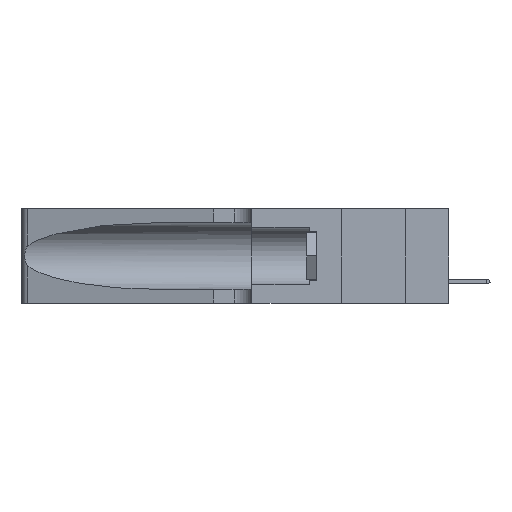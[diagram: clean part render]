
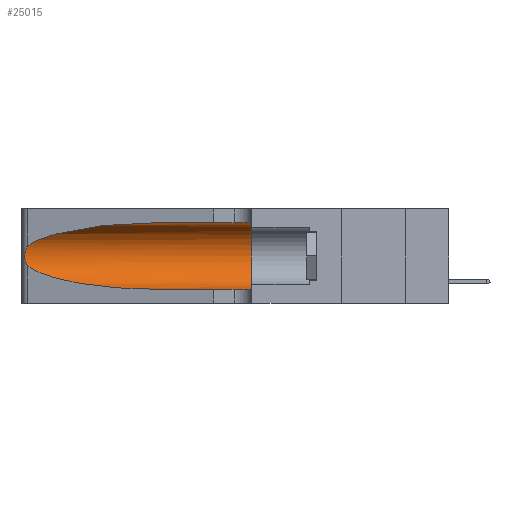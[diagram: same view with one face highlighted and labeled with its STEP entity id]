
A CAD part, left-side view. The second image highlights one B-rep face of the part: STEP entity #25015.
In plain terms, the highlighted cylindrical face has radius 3.308 mm (diameter 6.617 mm), a partial arc.
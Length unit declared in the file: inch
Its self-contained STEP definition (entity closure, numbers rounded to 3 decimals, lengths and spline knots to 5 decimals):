
#1150 = CARTESIAN_POINT ( 'NONE',  ( 0.25639, 1.23186, 0.15144 ) ) ;
#1614 = CARTESIAN_POINT ( 'NONE',  ( 0.25789, 1.23486, 0.15765 ) ) ;
#3197 = VERTEX_POINT ( 'NONE', #30987 ) ;
#4556 = CARTESIAN_POINT ( 'NONE',  ( 0.25639, 1.23184, 0.21858 ) ) ;
#4716 = CARTESIAN_POINT ( 'NONE',  ( 0.25487, 1.22718, 0.22369 ) ) ;
#4862 = CARTESIAN_POINT ( 'NONE',  ( 0.25854, 1.2359, 0.20912 ) ) ;
#5605 = ORIENTED_EDGE ( 'NONE', *, *, #19120, .T. ) ;
#5945 = ORIENTED_EDGE ( 'NONE', *, *, #38050, .T. ) ;
#5971 = EDGE_CURVE ( 'NONE', #21398, #3197, #44074, .T. ) ;
#7481 = EDGE_CURVE ( 'NONE', #19406, #3197, #38464, .T. ) ;
#7937 = CARTESIAN_POINT ( 'NONE',  ( 0.1305, 0.35, 0.31525 ) ) ;
#8434 = CARTESIAN_POINT ( 'NONE',  ( 0.26075, 1.23896, 0.19203 ) ) ;
#8736 = CARTESIAN_POINT ( 'NONE',  ( 0.25487, 1.22718, 0.14631 ) ) ;
#9208 = CARTESIAN_POINT ( 'NONE',  ( 0.25487, 1.22718, 0.22369 ) ) ;
#9624 = DIRECTION ( 'NONE',  ( 0., 0., 1. ) ) ;
#11632 = CARTESIAN_POINT ( 'NONE',  ( 0.1305, 0.72297, 0.31525 ) ) ;
#12654 = DIRECTION ( 'NONE',  ( 0., 0., -1. ) ) ;
#13403 = AXIS2_PLACEMENT_3D ( 'NONE', #30616, #40782, #9624 ) ;
#16372 = CARTESIAN_POINT ( 'NONE',  ( 0.1305, 1.61858, 0.05475 ) ) ;
#17282 = CARTESIAN_POINT ( 'NONE',  ( 0.2373, 1.15595, 0.28018 ) ) ;
#17976 = CARTESIAN_POINT ( 'NONE',  ( 0.1305, 1.61858, 0.31525 ) ) ;
#18551 = VECTOR ( 'NONE', #30289, 39.37008 ) ;
#19120 = EDGE_CURVE ( 'NONE', #34291, #19406, #44472, .T. ) ;
#19217 = CARTESIAN_POINT ( 'NONE',  ( 0.26017, 1.23833, 0.17102 ) ) ;
#19406 = VERTEX_POINT ( 'NONE', #29767 ) ;
#19437 = CARTESIAN_POINT ( 'NONE',  ( 0.18966, 0.96281, 0.05475 ) ) ;
#20327 = DIRECTION ( 'NONE',  ( 0., -1., 0. ) ) ;
#21398 = VERTEX_POINT ( 'NONE', #7937 ) ;
#21823 = EDGE_CURVE ( 'NONE', #23246, #34291, #42988, .T. ) ;
#22641 = CARTESIAN_POINT ( 'NONE',  ( 0.25555, 1.22994, 0.2215 ) ) ;
#22698 = CARTESIAN_POINT ( 'NONE',  ( 0.1305, 0.72297, 0.05475 ) ) ;
#22807 = CARTESIAN_POINT ( 'NONE',  ( 0.25856, 1.23593, 0.16098 ) ) ;
#23246 = VERTEX_POINT ( 'NONE', #9208 ) ;
#25015 = ADVANCED_FACE ( 'NONE', ( #35313 ), #33100, .F. ) ;
#26240 = CARTESIAN_POINT ( 'NONE',  ( 0.25487, 1.22718, 0.14631 ) ) ;
#26338 = CARTESIAN_POINT ( 'NONE',  ( 0.25555, 1.22993, 0.14849 ) ) ;
#26874 = CARTESIAN_POINT ( 'NONE',  ( 0.2373, 1.15595, 0.08982 ) ) ;
#27205 = CARTESIAN_POINT ( 'NONE',  ( 0.1305, 1.61858, 0.185 ) ) ;
#27216 = VERTEX_POINT ( 'NONE', #11632 ) ;
#28097 = CARTESIAN_POINT ( 'NONE',  ( 0.25487, 1.22718, 0.22369 ) ) ;
#29767 = CARTESIAN_POINT ( 'NONE',  ( 0.1305, 0.72297, 0.05475 ) ) ;
#30289 = DIRECTION ( 'NONE',  ( 0., -1., 0. ) ) ;
#30616 = CARTESIAN_POINT ( 'NONE',  ( 0.1305, 0.35, 0.185 ) ) ;
#30975 = ORIENTED_EDGE ( 'NONE', *, *, #7481, .T. ) ;
#30987 = CARTESIAN_POINT ( 'NONE',  ( 0.1305, 0.35, 0.05475 ) ) ;
#31242 = EDGE_CURVE ( 'NONE', #27216, #21398, #35997, .T. ) ;
#31627 = VECTOR ( 'NONE', #20327, 39.37008 ) ;
#32450 = ORIENTED_EDGE ( 'NONE', *, *, #5971, .F. ) ;
#32777 = CARTESIAN_POINT ( 'NONE',  ( 0.26018, 1.23835, 0.19895 ) ) ;
#32811 =( BOUNDED_CURVE ( )  B_SPLINE_CURVE ( 3, ( #45694, #42405, #17282, #28097 ),
 .UNSPECIFIED., .F., .F. ) 
 B_SPLINE_CURVE_WITH_KNOTS ( ( 4, 4 ),
 ( 1.5708, 2.84003 ),
 .UNSPECIFIED. ) 
 CURVE ( )  GEOMETRIC_REPRESENTATION_ITEM ( )  RATIONAL_B_SPLINE_CURVE ( ( 1., 0.87, 0.87, 1. ) ) 
 REPRESENTATION_ITEM ( '' )  );
#33100 = CYLINDRICAL_SURFACE ( 'NONE', #37695, 0.13025 ) ;
#34291 = VERTEX_POINT ( 'NONE', #36008 ) ;
#35313 = FACE_OUTER_BOUND ( 'NONE', #42453, .T. ) ;
#35997 = LINE ( 'NONE', #17976, #31627 ) ;
#36008 = CARTESIAN_POINT ( 'NONE',  ( 0.25487, 1.22718, 0.14631 ) ) ;
#36603 = ORIENTED_EDGE ( 'NONE', *, *, #21823, .T. ) ;
#37695 = AXIS2_PLACEMENT_3D ( 'NONE', #27205, #41205, #12654 ) ;
#38050 = EDGE_CURVE ( 'NONE', #27216, #23246, #32811, .T. ) ;
#38464 = LINE ( 'NONE', #16372, #18551 ) ;
#38467 = ORIENTED_EDGE ( 'NONE', *, *, #31242, .F. ) ;
#39886 = CARTESIAN_POINT ( 'NONE',  ( 0.25787, 1.23484, 0.2124 ) ) ;
#40358 = CARTESIAN_POINT ( 'NONE',  ( 0.26075, 1.23896, 0.178 ) ) ;
#40782 = DIRECTION ( 'NONE',  ( 0., 1., 0. ) ) ;
#41205 = DIRECTION ( 'NONE',  ( 0., -1., 0. ) ) ;
#42405 = CARTESIAN_POINT ( 'NONE',  ( 0.18966, 0.96281, 0.31525 ) ) ;
#42453 = EDGE_LOOP ( 'NONE', ( #5945, #36603, #5605, #30975, #32450, #38467 ) ) ;
#42988 = B_SPLINE_CURVE_WITH_KNOTS ( 'NONE', 3,
 ( #4716, #22641, #4556, #39886, #4862, #32777, #8434, #40358, #19217, #22807, #1614, #1150, #26338, #8736 ),
 .UNSPECIFIED., .F., .F.,
 ( 4, 2, 2, 2, 2, 2, 4 ),
 ( 0., 0.00027, 0.00053, 0.00107, 0.0016, 0.00187, 0.00214 ),
 .UNSPECIFIED. ) ;
#44074 = CIRCLE ( 'NONE', #13403, 0.13025 ) ;
#44472 =( BOUNDED_CURVE ( )  B_SPLINE_CURVE ( 3, ( #26240, #26874, #19437, #22698 ),
 .UNSPECIFIED., .F., .T. ) 
 B_SPLINE_CURVE_WITH_KNOTS ( ( 4, 4 ),
 ( 3.44316, 4.71239 ),
 .UNSPECIFIED. ) 
 CURVE ( )  GEOMETRIC_REPRESENTATION_ITEM ( )  RATIONAL_B_SPLINE_CURVE ( ( 1., 0.87, 0.87, 1. ) ) 
 REPRESENTATION_ITEM ( '' )  );
#45694 = CARTESIAN_POINT ( 'NONE',  ( 0.1305, 0.72297, 0.31525 ) ) ;
